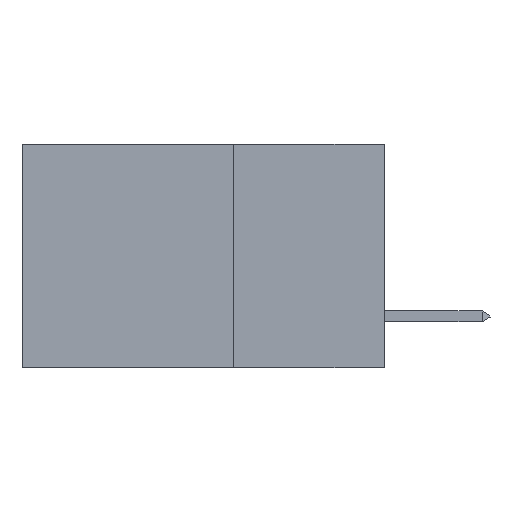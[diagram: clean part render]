
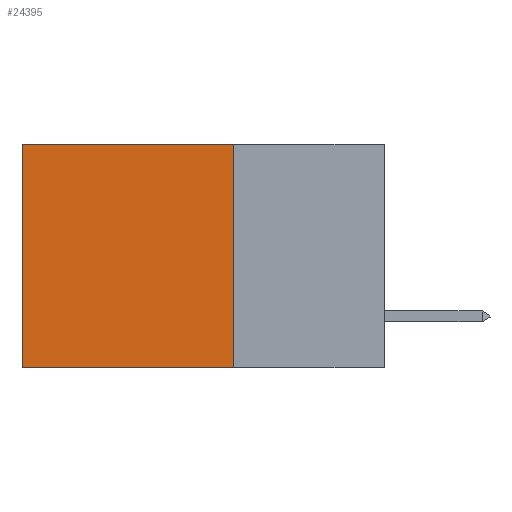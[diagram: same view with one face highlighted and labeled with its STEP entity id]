
A CAD part, left-side view. The second image highlights one B-rep face of the part: STEP entity #24395.
In plain terms, the highlighted planar face has unit normal (-1, 0, 0).
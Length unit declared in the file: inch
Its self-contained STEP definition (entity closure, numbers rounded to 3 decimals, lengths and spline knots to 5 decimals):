
#1163 = DIRECTION ( 'NONE',  ( 1., 0., 0. ) ) ;
#1601 = PLANE ( 'NONE',  #1604 ) ;
#1604 = AXIS2_PLACEMENT_3D ( 'NONE', #18495, #1163, #24875 ) ;
#2347 = VECTOR ( 'NONE', #19507, 39.37008 ) ;
#3767 = CARTESIAN_POINT ( 'NONE',  ( 0.2875, 0.6, -0.37 ) ) ;
#4606 = FACE_OUTER_BOUND ( 'NONE', #9833, .T. ) ;
#6898 = VERTEX_POINT ( 'NONE', #26330 ) ;
#6910 = CARTESIAN_POINT ( 'NONE',  ( 0.2875, 0.25, 0. ) ) ;
#9833 = EDGE_LOOP ( 'NONE', ( #30349, #27622, #21359, #13272 ) ) ;
#11676 = CARTESIAN_POINT ( 'NONE',  ( 0.2875, 0.25, 0. ) ) ;
#13272 = ORIENTED_EDGE ( 'NONE', *, *, #20302, .T. ) ;
#14572 = LINE ( 'NONE', #39741, #2347 ) ;
#15359 = LINE ( 'NONE', #6910, #23298 ) ;
#16952 = VERTEX_POINT ( 'NONE', #20955 ) ;
#18495 = CARTESIAN_POINT ( 'NONE',  ( 0.2875, 0.25, 0. ) ) ;
#19507 = DIRECTION ( 'NONE',  ( 0., 1., 0. ) ) ;
#20302 = EDGE_CURVE ( 'NONE', #30674, #16952, #14572, .T. ) ;
#20814 = VECTOR ( 'NONE', #43046, 39.37008 ) ;
#20955 = CARTESIAN_POINT ( 'NONE',  ( 0.2875, 0.6, 0. ) ) ;
#21359 = ORIENTED_EDGE ( 'NONE', *, *, #22871, .F. ) ;
#22871 = EDGE_CURVE ( 'NONE', #30674, #6898, #15359, .T. ) ;
#23298 = VECTOR ( 'NONE', #30673, 39.37008 ) ;
#23488 = DIRECTION ( 'NONE',  ( 0., 0., -1. ) ) ;
#24395 = ADVANCED_FACE ( 'NONE', ( #4606 ), #1601, .F. ) ;
#24492 = LINE ( 'NONE', #42033, #20814 ) ;
#24875 = DIRECTION ( 'NONE',  ( 0., 0., -1. ) ) ;
#26330 = CARTESIAN_POINT ( 'NONE',  ( 0.2875, 0.25, -0.37 ) ) ;
#27622 = ORIENTED_EDGE ( 'NONE', *, *, #42641, .F. ) ;
#30349 = ORIENTED_EDGE ( 'NONE', *, *, #40428, .T. ) ;
#30673 = DIRECTION ( 'NONE',  ( 0., 0., -1. ) ) ;
#30674 = VERTEX_POINT ( 'NONE', #11676 ) ;
#39741 = CARTESIAN_POINT ( 'NONE',  ( 0.2875, 0.25, 0. ) ) ;
#40037 = CARTESIAN_POINT ( 'NONE',  ( 0.2875, 0.6, 0. ) ) ;
#40428 = EDGE_CURVE ( 'NONE', #16952, #41700, #43946, .T. ) ;
#41282 = VECTOR ( 'NONE', #23488, 39.37008 ) ;
#41700 = VERTEX_POINT ( 'NONE', #3767 ) ;
#42033 = CARTESIAN_POINT ( 'NONE',  ( 0.2875, 0.25, -0.37 ) ) ;
#42641 = EDGE_CURVE ( 'NONE', #6898, #41700, #24492, .T. ) ;
#43046 = DIRECTION ( 'NONE',  ( 0., 1., 0. ) ) ;
#43946 = LINE ( 'NONE', #40037, #41282 ) ;
